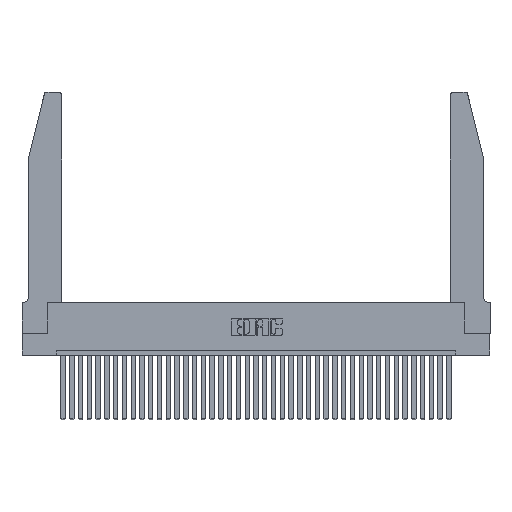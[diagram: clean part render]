
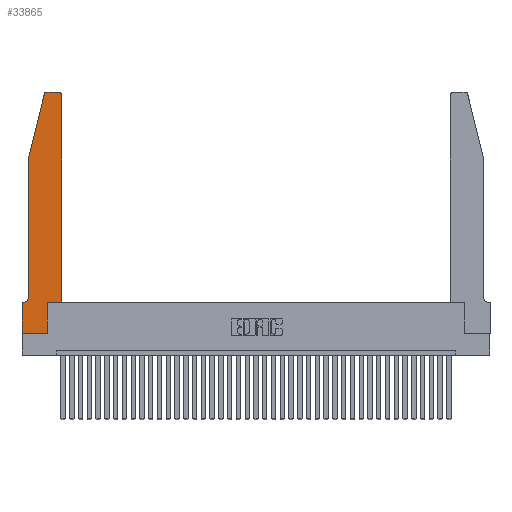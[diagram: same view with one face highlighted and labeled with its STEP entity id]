
A CAD part, top view. The second image highlights one B-rep face of the part: STEP entity #33865.
In plain terms, the highlighted planar face has unit normal (0, 0, 1).
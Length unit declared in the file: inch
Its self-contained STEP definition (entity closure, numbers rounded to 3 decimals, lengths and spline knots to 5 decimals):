
#422 = AXIS2_PLACEMENT_3D ( 'NONE', #1120, #10127, #7276 ) ;
#830 = DIRECTION ( 'NONE',  ( -1., 0., 0. ) ) ;
#1088 = CARTESIAN_POINT ( 'NONE',  ( 0.0055, 0.42, 0.37 ) ) ;
#1120 = CARTESIAN_POINT ( 'NONE',  ( 0.284, 2.72, 0.37 ) ) ;
#1271 = CARTESIAN_POINT ( 'NONE',  ( 0.0755, 0.42, 0.37 ) ) ;
#1304 = DIRECTION ( 'NONE',  ( 1., 0., 0. ) ) ;
#1684 = DIRECTION ( 'NONE',  ( -1., 0., 0. ) ) ;
#2157 = ORIENTED_EDGE ( 'NONE', *, *, #25858, .T. ) ;
#2365 = VERTEX_POINT ( 'NONE', #29327 ) ;
#2450 = EDGE_CURVE ( 'NONE', #34541, #22417, #7481, .T. ) ;
#2618 = ORIENTED_EDGE ( 'NONE', *, *, #2450, .T. ) ;
#2766 = CARTESIAN_POINT ( 'NONE',  ( 0., 0., 0.37 ) ) ;
#3109 = EDGE_CURVE ( 'NONE', #35693, #34541, #24519, .T. ) ;
#3322 = LINE ( 'NONE', #23483, #5162 ) ;
#4796 = CARTESIAN_POINT ( 'NONE',  ( 0.2865, 0., 0.37 ) ) ;
#5162 = VECTOR ( 'NONE', #1304, 39.37008 ) ;
#5171 = EDGE_LOOP ( 'NONE', ( #8814, #36029, #2618, #29884, #25822, #27001, #29071, #35232, #2157, #22674, #33232, #29505 ) ) ;
#5313 = CARTESIAN_POINT ( 'NONE',  ( 0.4505, 0.35, 0.37 ) ) ;
#5566 = FACE_OUTER_BOUND ( 'NONE', #5171, .T. ) ;
#5790 = VERTEX_POINT ( 'NONE', #17885 ) ;
#6577 = LINE ( 'NONE', #34523, #18561 ) ;
#7276 = DIRECTION ( 'NONE',  ( 1., 0., 0. ) ) ;
#7481 = LINE ( 'NONE', #31363, #30053 ) ;
#7752 = CARTESIAN_POINT ( 'NONE',  ( 0.2865, 0.35, 0.37 ) ) ;
#8258 = CARTESIAN_POINT ( 'NONE',  ( 0., 0.35, 0.37 ) ) ;
#8565 = CARTESIAN_POINT ( 'NONE',  ( 0., 0.35, 0.37 ) ) ;
#8682 = CIRCLE ( 'NONE', #14100, 0.03 ) ;
#8814 = ORIENTED_EDGE ( 'NONE', *, *, #12838, .T. ) ;
#9593 = EDGE_CURVE ( 'NONE', #35587, #27683, #3322, .T. ) ;
#10127 = DIRECTION ( 'NONE',  ( 0., 0., 1. ) ) ;
#10185 = LINE ( 'NONE', #36986, #35938 ) ;
#10609 = CARTESIAN_POINT ( 'NONE',  ( 0.2865, 0.35, 0.37 ) ) ;
#11368 = DIRECTION ( 'NONE',  ( 0., 0., 1. ) ) ;
#12089 = VERTEX_POINT ( 'NONE', #4796 ) ;
#12451 = EDGE_CURVE ( 'NONE', #17249, #29085, #28807, .T. ) ;
#12788 = EDGE_CURVE ( 'NONE', #22417, #17249, #30132, .T. ) ;
#12838 = EDGE_CURVE ( 'NONE', #33388, #35693, #37906, .T. ) ;
#14100 = AXIS2_PLACEMENT_3D ( 'NONE', #35636, #26887, #14376 ) ;
#14376 = DIRECTION ( 'NONE',  ( 1., 0., 0. ) ) ;
#14501 = LINE ( 'NONE', #10609, #17739 ) ;
#14556 = DIRECTION ( 'NONE',  ( 0., 1., 0. ) ) ;
#14728 = DIRECTION ( 'NONE',  ( -1., 0., 0. ) ) ;
#16777 = CARTESIAN_POINT ( 'NONE',  ( 0.25487, 2.72718, 0.37 ) ) ;
#16830 = CARTESIAN_POINT ( 'NONE',  ( 0.0755, 2., 0.37 ) ) ;
#16848 = DIRECTION ( 'NONE',  ( -0.239, -0.971, 0. ) ) ;
#17083 = EDGE_CURVE ( 'NONE', #5790, #33388, #8682, .T. ) ;
#17249 = VERTEX_POINT ( 'NONE', #1271 ) ;
#17739 = VECTOR ( 'NONE', #36917, 39.37008 ) ;
#17885 = CARTESIAN_POINT ( 'NONE',  ( 0.4505, 2.72, 0.37 ) ) ;
#18561 = VECTOR ( 'NONE', #25401, 39.37008 ) ;
#19719 = AXIS2_PLACEMENT_3D ( 'NONE', #1088, #30565, #830 ) ;
#20140 = DIRECTION ( 'NONE',  ( 0., -1., 0. ) ) ;
#20426 = CARTESIAN_POINT ( 'NONE',  ( 0.2605, 2.75, 0.37 ) ) ;
#22361 = LINE ( 'NONE', #35252, #32044 ) ;
#22417 = VERTEX_POINT ( 'NONE', #16830 ) ;
#22590 = AXIS2_PLACEMENT_3D ( 'NONE', #8258, #11368, #31703 ) ;
#22674 = ORIENTED_EDGE ( 'NONE', *, *, #9593, .T. ) ;
#22849 = CARTESIAN_POINT ( 'NONE',  ( 0.284, 2.75, 0.37 ) ) ;
#23483 = CARTESIAN_POINT ( 'NONE',  ( 0.4505, 0.35, 0.37 ) ) ;
#24519 = CIRCLE ( 'NONE', #422, 0.03 ) ;
#25079 = VECTOR ( 'NONE', #29403, 39.37008 ) ;
#25401 = DIRECTION ( 'NONE',  ( 1., 0., 0. ) ) ;
#25583 = CARTESIAN_POINT ( 'NONE',  ( 0.4205, 2.75, 0.37 ) ) ;
#25822 = ORIENTED_EDGE ( 'NONE', *, *, #12451, .T. ) ;
#25858 = EDGE_CURVE ( 'NONE', #12089, #35587, #14501, .T. ) ;
#25924 = PLANE ( 'NONE',  #22590 ) ;
#26019 = VECTOR ( 'NONE', #14728, 39.37008 ) ;
#26887 = DIRECTION ( 'NONE',  ( 0., 0., 1. ) ) ;
#26960 = EDGE_CURVE ( 'NONE', #2365, #12089, #6577, .T. ) ;
#27001 = ORIENTED_EDGE ( 'NONE', *, *, #33225, .T. ) ;
#27065 = CARTESIAN_POINT ( 'NONE',  ( 0.0055, 0.35, 0.37 ) ) ;
#27683 = VERTEX_POINT ( 'NONE', #5313 ) ;
#28743 = CARTESIAN_POINT ( 'NONE',  ( 0.0755, 2., 0.37 ) ) ;
#28807 = CIRCLE ( 'NONE', #19719, 0.07 ) ;
#29071 = ORIENTED_EDGE ( 'NONE', *, *, #31878, .T. ) ;
#29085 = VERTEX_POINT ( 'NONE', #27065 ) ;
#29327 = CARTESIAN_POINT ( 'NONE',  ( 0., 0., 0.37 ) ) ;
#29403 = DIRECTION ( 'NONE',  ( 0., -1., 0. ) ) ;
#29505 = ORIENTED_EDGE ( 'NONE', *, *, #17083, .T. ) ;
#29884 = ORIENTED_EDGE ( 'NONE', *, *, #12788, .T. ) ;
#30053 = VECTOR ( 'NONE', #16848, 39.37008 ) ;
#30132 = LINE ( 'NONE', #28743, #25079 ) ;
#30565 = DIRECTION ( 'NONE',  ( 0., 0., -1. ) ) ;
#31363 = CARTESIAN_POINT ( 'NONE',  ( 0.0755, 2., 0.37 ) ) ;
#31703 = DIRECTION ( 'NONE',  ( 1., 0., 0. ) ) ;
#31878 = EDGE_CURVE ( 'NONE', #35094, #2365, #37816, .T. ) ;
#32044 = VECTOR ( 'NONE', #14556, 39.37008 ) ;
#32334 = VECTOR ( 'NONE', #20140, 39.37008 ) ;
#33225 = EDGE_CURVE ( 'NONE', #29085, #35094, #10185, .T. ) ;
#33232 = ORIENTED_EDGE ( 'NONE', *, *, #36299, .T. ) ;
#33388 = VERTEX_POINT ( 'NONE', #25583 ) ;
#33865 = ADVANCED_FACE ( 'NONE', ( #5566 ), #25924, .T. ) ;
#34523 = CARTESIAN_POINT ( 'NONE',  ( 0., 0., 0.37 ) ) ;
#34541 = VERTEX_POINT ( 'NONE', #16777 ) ;
#35094 = VERTEX_POINT ( 'NONE', #8565 ) ;
#35232 = ORIENTED_EDGE ( 'NONE', *, *, #26960, .T. ) ;
#35252 = CARTESIAN_POINT ( 'NONE',  ( 0.4505, 0.35, 0.37 ) ) ;
#35587 = VERTEX_POINT ( 'NONE', #7752 ) ;
#35636 = CARTESIAN_POINT ( 'NONE',  ( 0.4205, 2.72, 0.37 ) ) ;
#35693 = VERTEX_POINT ( 'NONE', #22849 ) ;
#35938 = VECTOR ( 'NONE', #1684, 39.37008 ) ;
#36029 = ORIENTED_EDGE ( 'NONE', *, *, #3109, .T. ) ;
#36299 = EDGE_CURVE ( 'NONE', #27683, #5790, #22361, .T. ) ;
#36917 = DIRECTION ( 'NONE',  ( 0., 1., 0. ) ) ;
#36986 = CARTESIAN_POINT ( 'NONE',  ( 0.0755, 0.35, 0.37 ) ) ;
#37816 = LINE ( 'NONE', #2766, #32334 ) ;
#37906 = LINE ( 'NONE', #20426, #26019 ) ;
